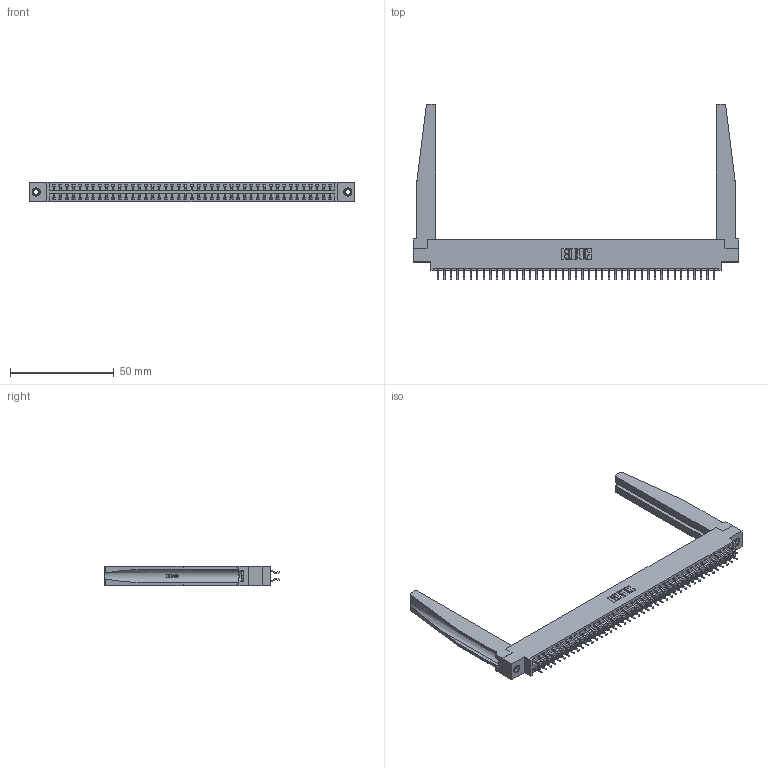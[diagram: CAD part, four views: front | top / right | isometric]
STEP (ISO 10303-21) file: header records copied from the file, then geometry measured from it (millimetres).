
FILE_DESCRIPTION (( 'STEP AP203' ), '1' );
FILE_NAME ('346-086-556-878.STEP', '2022-05-25T23:16:47', ( '' ), ( '' ), 'SwSTEP 2.0', 'SolidWorks 2020', '' );
FILE_SCHEMA (( 'CONFIG_CONTROL_DESIGN' ));
Length unit declared in the file: inch
Products named in the file (5): 346-086-556-878; 345-250-001_345-250-001-102; 345-292-001_556 Tail; 346 Part_0.170 Offset - 0.156 Dia-TH; 346-220-078_345-220-078
Assembly tree (91 placements, depth 2):
  346-086-556-878
    346 Part_0.170 Offset - 0.156 Dia-TH
    345-292-001_556 Tail  x86
    346-220-078_345-220-078  x2
    345-250-001_345-250-001-102  x2
Bounding box: 157.1 x 84.84 x 9.4 mm (x, y, z)
Volume: 22059.6 mm3; surface area: 27513.2 mm2
Topology: 91 solids, 91 shells, 5362 faces, 15863 edges, 10450 vertices
Faces by surface type: plane 3590, cylinder 1720, bspline 36, cone 12, torus 4
Entity records: 33444 total; most frequent: CARTESIAN_POINT 6469, ORIENTED_EDGE 5278, DIRECTION 4725, EDGE_CURVE 2639, LINE 2233, VECTOR 2233, VERTEX_POINT 1752, AXIS2_PLACEMENT_3D 1246
